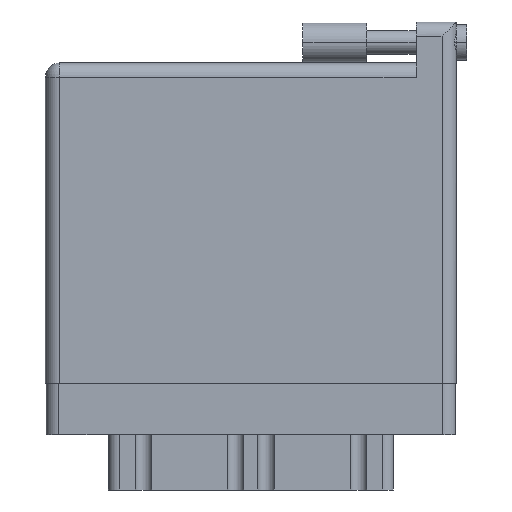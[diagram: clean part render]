
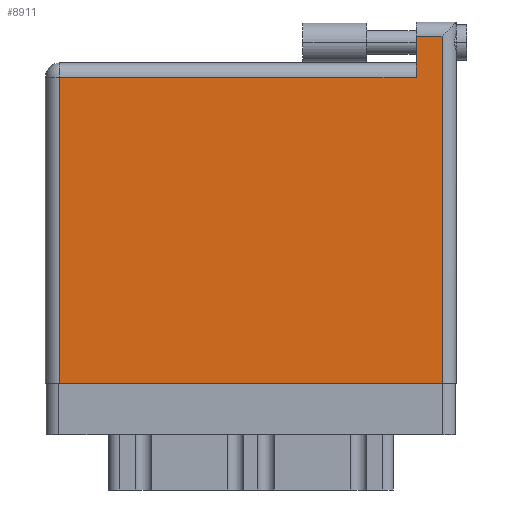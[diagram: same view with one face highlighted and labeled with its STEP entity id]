
A CAD part, front view. The second image highlights one B-rep face of the part: STEP entity #8911.
In plain terms, the highlighted face is planar.
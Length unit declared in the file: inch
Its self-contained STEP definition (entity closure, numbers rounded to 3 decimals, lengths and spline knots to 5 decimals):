
#2422 = ORIENTED_EDGE ( 'NONE', *, *, #7586, .T. ) ;
#3586 = EDGE_CURVE ( 'NONE', #13665, #11446, #24829, .T. ) ;
#3791 = PLANE ( 'NONE',  #26115 ) ;
#4039 = DIRECTION ( 'NONE',  ( -1., 0., 0. ) ) ;
#4470 = VERTEX_POINT ( 'NONE', #6587 ) ;
#6587 = CARTESIAN_POINT ( 'NONE',  ( 1.938, 1.696, 0. ) ) ;
#7586 = EDGE_CURVE ( 'NONE', #7998, #13665, #11704, .T. ) ;
#7998 = VERTEX_POINT ( 'NONE', #19346 ) ;
#8136 = ORIENTED_EDGE ( 'NONE', *, *, #9534, .T. ) ;
#8429 = FACE_OUTER_BOUND ( 'NONE', #16945, .T. ) ;
#8541 = DIRECTION ( 'NONE',  ( 0., 1., 0. ) ) ;
#8774 = VECTOR ( 'NONE', #21296, 39.37008 ) ;
#8886 = VECTOR ( 'NONE', #17383, 39.37008 ) ;
#8911 = ADVANCED_FACE ( 'NONE', ( #8429 ), #3791, .F. ) ;
#9532 = ORIENTED_EDGE ( 'NONE', *, *, #3586, .T. ) ;
#9534 = EDGE_CURVE ( 'NONE', #4470, #24762, #13781, .T. ) ;
#10885 = CARTESIAN_POINT ( 'NONE',  ( 1.811, 1.696, 0. ) ) ;
#11446 = VERTEX_POINT ( 'NONE', #13422 ) ;
#11508 = DIRECTION ( 'NONE',  ( 0., -1., 0. ) ) ;
#11704 = LINE ( 'NONE', #21144, #8774 ) ;
#12580 = VECTOR ( 'NONE', #4039, 39.37008 ) ;
#12778 = DIRECTION ( 'NONE',  ( -1., 0., 0. ) ) ;
#13327 = EDGE_CURVE ( 'NONE', #17171, #7998, #26692, .T. ) ;
#13422 = CARTESIAN_POINT ( 'NONE',  ( 1.938, 0., 0. ) ) ;
#13529 = LINE ( 'NONE', #16001, #29668 ) ;
#13665 = VERTEX_POINT ( 'NONE', #15978 ) ;
#13781 = LINE ( 'NONE', #30355, #30569 ) ;
#13938 = DIRECTION ( 'NONE',  ( -1., 0., 0. ) ) ;
#15799 = CARTESIAN_POINT ( 'NONE',  ( 0., 1.496, 0. ) ) ;
#15978 = CARTESIAN_POINT ( 'NONE',  ( 0.07, 0., 0. ) ) ;
#16001 = CARTESIAN_POINT ( 'NONE',  ( 1.811, 1.766, 0. ) ) ;
#16945 = EDGE_LOOP ( 'NONE', ( #9532, #17817, #8136, #27215, #30144, #2422 ) ) ;
#17171 = VERTEX_POINT ( 'NONE', #29366 ) ;
#17383 = DIRECTION ( 'NONE',  ( 1., 0., 0. ) ) ;
#17817 = ORIENTED_EDGE ( 'NONE', *, *, #20175, .T. ) ;
#18591 = CARTESIAN_POINT ( 'NONE',  ( 1.938, 1.766, 0. ) ) ;
#19346 = CARTESIAN_POINT ( 'NONE',  ( 0.07, 1.496, 0. ) ) ;
#19849 = EDGE_CURVE ( 'NONE', #24762, #17171, #13529, .T. ) ;
#20175 = EDGE_CURVE ( 'NONE', #11446, #4470, #30368, .T. ) ;
#20323 = CARTESIAN_POINT ( 'NONE',  ( 0., 0., 0. ) ) ;
#21144 = CARTESIAN_POINT ( 'NONE',  ( 0.07, 0., 0. ) ) ;
#21296 = DIRECTION ( 'NONE',  ( 0., -1., 0. ) ) ;
#22069 = CARTESIAN_POINT ( 'NONE',  ( 0., 1.566, 0. ) ) ;
#24687 = VECTOR ( 'NONE', #8541, 39.37008 ) ;
#24762 = VERTEX_POINT ( 'NONE', #10885 ) ;
#24829 = LINE ( 'NONE', #20323, #8886 ) ;
#25013 = DIRECTION ( 'NONE',  ( 0., 0., -1. ) ) ;
#26115 = AXIS2_PLACEMENT_3D ( 'NONE', #22069, #25013, #12778 ) ;
#26692 = LINE ( 'NONE', #15799, #12580 ) ;
#27215 = ORIENTED_EDGE ( 'NONE', *, *, #19849, .T. ) ;
#29366 = CARTESIAN_POINT ( 'NONE',  ( 1.811, 1.496, 0. ) ) ;
#29668 = VECTOR ( 'NONE', #11508, 39.37008 ) ;
#30144 = ORIENTED_EDGE ( 'NONE', *, *, #13327, .T. ) ;
#30355 = CARTESIAN_POINT ( 'NONE',  ( 0., 1.696, 0. ) ) ;
#30368 = LINE ( 'NONE', #18591, #24687 ) ;
#30569 = VECTOR ( 'NONE', #13938, 39.37008 ) ;
